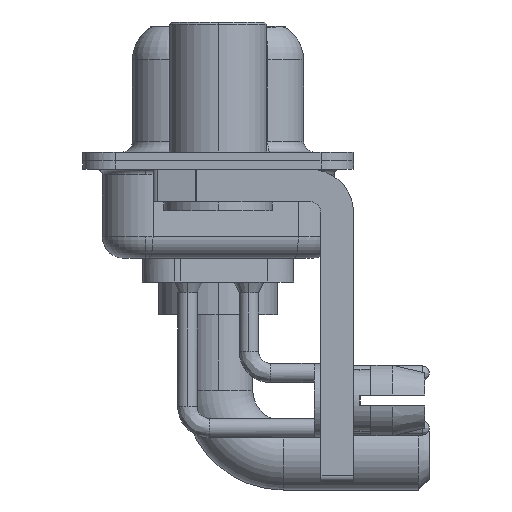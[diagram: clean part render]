
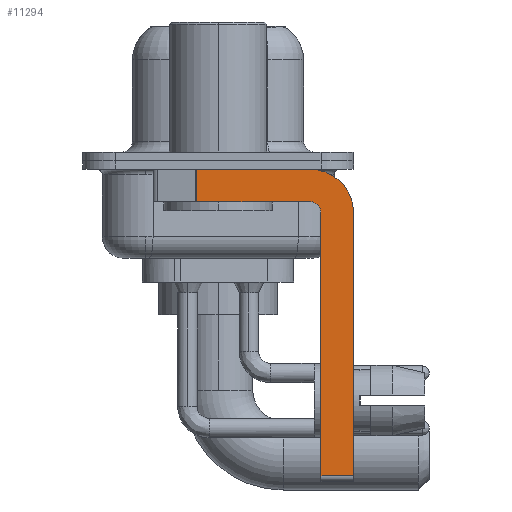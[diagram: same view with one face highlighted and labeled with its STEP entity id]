
A CAD part, left-side view. The second image highlights one B-rep face of the part: STEP entity #11294.
In plain terms, the highlighted planar face has unit normal (-1, 0, 0).
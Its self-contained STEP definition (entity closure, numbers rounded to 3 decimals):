
#48 = VERTEX_POINT ( 'NONE', #15521 ) ;
#1405 = CARTESIAN_POINT ( 'NONE',  ( -2.9, 0.978, -1.9 ) ) ;
#1690 = ORIENTED_EDGE ( 'NONE', *, *, #20069, .F. ) ;
#1964 = CARTESIAN_POINT ( 'NONE',  ( -2.9, -4.75, -2.4 ) ) ;
#2024 = LINE ( 'NONE', #21314, #5074 ) ;
#2354 = CIRCLE ( 'NONE', #5268, 0.5 ) ;
#2604 = DIRECTION ( 'NONE',  ( 0., 0., -1. ) ) ;
#2627 = CARTESIAN_POINT ( 'NONE',  ( -2.9, -6.25, -14.55 ) ) ;
#2643 = ORIENTED_EDGE ( 'NONE', *, *, #22388, .F. ) ;
#2867 = CARTESIAN_POINT ( 'NONE',  ( -2.9, -4.25, -2.4 ) ) ;
#2943 = VERTEX_POINT ( 'NONE', #1964 ) ;
#2975 = CARTESIAN_POINT ( 'NONE',  ( -2.9, -4.75, -14.8 ) ) ;
#3771 = ORIENTED_EDGE ( 'NONE', *, *, #8049, .F. ) ;
#4670 = DIRECTION ( 'NONE',  ( -1., 0., 0. ) ) ;
#4794 = CARTESIAN_POINT ( 'NONE',  ( -2.9, -4.25, -14.55 ) ) ;
#4962 = LINE ( 'NONE', #8510, #12852 ) ;
#5074 = VECTOR ( 'NONE', #12545, 1000. ) ;
#5268 = AXIS2_PLACEMENT_3D ( 'NONE', #20301, #4670, #19967 ) ;
#5382 = CARTESIAN_POINT ( 'NONE',  ( -2.9, -4.75, -14.55 ) ) ;
#5936 = VERTEX_POINT ( 'NONE', #2627 ) ;
#5975 = EDGE_CURVE ( 'NONE', #13630, #12296, #17216, .T. ) ;
#6106 = EDGE_CURVE ( 'NONE', #10102, #5936, #17115, .T. ) ;
#6471 = ORIENTED_EDGE ( 'NONE', *, *, #6106, .T. ) ;
#6610 = VERTEX_POINT ( 'NONE', #14006 ) ;
#6981 = VECTOR ( 'NONE', #2604, 1000. ) ;
#7900 = ORIENTED_EDGE ( 'NONE', *, *, #19799, .F. ) ;
#8049 = EDGE_CURVE ( 'NONE', #2943, #48, #2354, .T. ) ;
#8134 = DIRECTION ( 'NONE',  ( 0., 0., -1. ) ) ;
#8510 = CARTESIAN_POINT ( 'NONE',  ( -2.9, -4.25, -1.9 ) ) ;
#8985 = AXIS2_PLACEMENT_3D ( 'NONE', #2867, #13391, #8134 ) ;
#10102 = VERTEX_POINT ( 'NONE', #5382 ) ;
#10296 = DIRECTION ( 'NONE',  ( 0., 0., 1. ) ) ;
#10314 = AXIS2_PLACEMENT_3D ( 'NONE', #22355, #15281, #18831 ) ;
#11288 = CARTESIAN_POINT ( 'NONE',  ( -2.9, -6.25, -2.4 ) ) ;
#11294 = ADVANCED_FACE ( 'NONE', ( #18507 ), #16685, .F. ) ;
#11471 = ORIENTED_EDGE ( 'NONE', *, *, #18841, .F. ) ;
#12296 = VERTEX_POINT ( 'NONE', #22319 ) ;
#12545 = DIRECTION ( 'NONE',  ( 0., 0., -1. ) ) ;
#12713 = ORIENTED_EDGE ( 'NONE', *, *, #12895, .T. ) ;
#12852 = VECTOR ( 'NONE', #20366, 1000. ) ;
#12895 = EDGE_CURVE ( 'NONE', #6610, #13468, #2024, .T. ) ;
#13391 = DIRECTION ( 'NONE',  ( 1., 0., 0. ) ) ;
#13468 = VERTEX_POINT ( 'NONE', #1405 ) ;
#13630 = VERTEX_POINT ( 'NONE', #16812 ) ;
#14006 = CARTESIAN_POINT ( 'NONE',  ( -2.9, 0.978, -0.4 ) ) ;
#15259 = LINE ( 'NONE', #22215, #22231 ) ;
#15281 = DIRECTION ( 'NONE',  ( 1., 0., 0. ) ) ;
#15521 = CARTESIAN_POINT ( 'NONE',  ( -2.9, -4.25, -1.9 ) ) ;
#16197 = LINE ( 'NONE', #11288, #6981 ) ;
#16685 = PLANE ( 'NONE',  #8985 ) ;
#16812 = CARTESIAN_POINT ( 'NONE',  ( -2.9, -4.25, -0.4 ) ) ;
#17115 = LINE ( 'NONE', #4794, #20875 ) ;
#17205 = DIRECTION ( 'NONE',  ( 0., -1., 0. ) ) ;
#17216 = CIRCLE ( 'NONE', #10314, 2. ) ;
#17271 = EDGE_LOOP ( 'NONE', ( #11471, #12713, #2643, #3771, #7900, #6471, #1690, #17332 ) ) ;
#17332 = ORIENTED_EDGE ( 'NONE', *, *, #5975, .F. ) ;
#18246 = VECTOR ( 'NONE', #10296, 1000. ) ;
#18507 = FACE_OUTER_BOUND ( 'NONE', #17271, .T. ) ;
#18831 = DIRECTION ( 'NONE',  ( 0., 0., -1. ) ) ;
#18841 = EDGE_CURVE ( 'NONE', #6610, #13630, #15259, .T. ) ;
#18937 = DIRECTION ( 'NONE',  ( 0., -1., 0. ) ) ;
#18946 = LINE ( 'NONE', #2975, #18246 ) ;
#19799 = EDGE_CURVE ( 'NONE', #10102, #2943, #18946, .T. ) ;
#19967 = DIRECTION ( 'NONE',  ( 0., 0., 1. ) ) ;
#20069 = EDGE_CURVE ( 'NONE', #12296, #5936, #16197, .T. ) ;
#20301 = CARTESIAN_POINT ( 'NONE',  ( -2.9, -4.25, -2.4 ) ) ;
#20366 = DIRECTION ( 'NONE',  ( 0., 1., 0. ) ) ;
#20875 = VECTOR ( 'NONE', #18937, 1000. ) ;
#21314 = CARTESIAN_POINT ( 'NONE',  ( -2.9, 0.978, -1.9 ) ) ;
#22215 = CARTESIAN_POINT ( 'NONE',  ( -2.9, 3., -0.4 ) ) ;
#22231 = VECTOR ( 'NONE', #17205, 1000. ) ;
#22319 = CARTESIAN_POINT ( 'NONE',  ( -2.9, -6.25, -2.4 ) ) ;
#22355 = CARTESIAN_POINT ( 'NONE',  ( -2.9, -4.25, -2.4 ) ) ;
#22388 = EDGE_CURVE ( 'NONE', #48, #13468, #4962, .T. ) ;
